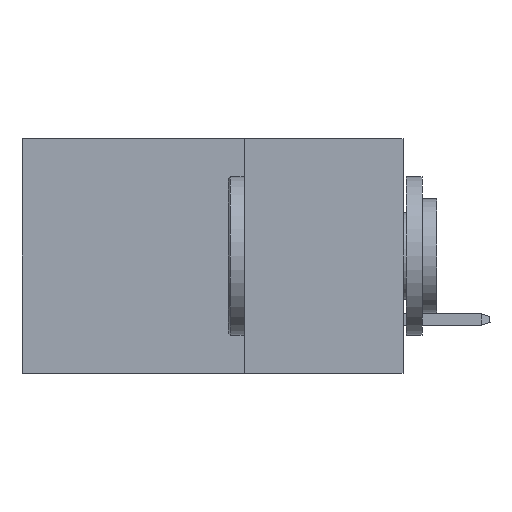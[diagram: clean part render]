
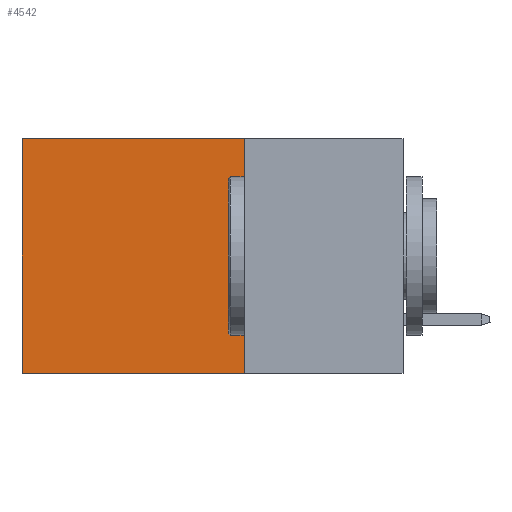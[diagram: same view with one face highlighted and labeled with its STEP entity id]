
A CAD part, left-side view. The second image highlights one B-rep face of the part: STEP entity #4542.
In plain terms, the highlighted planar face has unit normal (-1, 0, 0).
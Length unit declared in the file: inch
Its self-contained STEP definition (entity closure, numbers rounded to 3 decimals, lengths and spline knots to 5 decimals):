
#105 = VERTEX_POINT ( 'NONE', #7938 ) ;
#736 = CARTESIAN_POINT ( 'NONE',  ( 0.2875, 0.6, -0.37 ) ) ;
#773 = FACE_OUTER_BOUND ( 'NONE', #12620, .T. ) ;
#2806 = DIRECTION ( 'NONE',  ( 0., 1., 0. ) ) ;
#4542 = ADVANCED_FACE ( 'NONE', ( #773 ), #39157, .F. ) ;
#7938 = CARTESIAN_POINT ( 'NONE',  ( 0.2875, 0.25, -0.37 ) ) ;
#8342 = DIRECTION ( 'NONE',  ( 0., 0., -1. ) ) ;
#8519 = ORIENTED_EDGE ( 'NONE', *, *, #19342, .F. ) ;
#10536 = CARTESIAN_POINT ( 'NONE',  ( 0.2875, 0.25, 0. ) ) ;
#10607 = VECTOR ( 'NONE', #21859, 39.37008 ) ;
#10879 = VECTOR ( 'NONE', #2806, 39.37008 ) ;
#11262 = LINE ( 'NONE', #11458, #16919 ) ;
#11458 = CARTESIAN_POINT ( 'NONE',  ( 0.2875, 0.6, 0. ) ) ;
#12620 = EDGE_LOOP ( 'NONE', ( #39764, #29908, #8519, #24910 ) ) ;
#13743 = VERTEX_POINT ( 'NONE', #37082 ) ;
#15112 = EDGE_CURVE ( 'NONE', #27222, #13743, #31443, .T. ) ;
#15869 = EDGE_CURVE ( 'NONE', #13743, #30124, #11262, .T. ) ;
#16919 = VECTOR ( 'NONE', #8342, 39.37008 ) ;
#18236 = CARTESIAN_POINT ( 'NONE',  ( 0.2875, 0.25, 0. ) ) ;
#18391 = DIRECTION ( 'NONE',  ( 0., 0., -1. ) ) ;
#18647 = AXIS2_PLACEMENT_3D ( 'NONE', #10536, #32322, #23384 ) ;
#19342 = EDGE_CURVE ( 'NONE', #27222, #105, #33955, .T. ) ;
#21859 = DIRECTION ( 'NONE',  ( 0., 1., 0. ) ) ;
#22992 = VECTOR ( 'NONE', #18391, 39.37008 ) ;
#23158 = EDGE_CURVE ( 'NONE', #105, #30124, #37854, .T. ) ;
#23384 = DIRECTION ( 'NONE',  ( 0., 0., -1. ) ) ;
#24910 = ORIENTED_EDGE ( 'NONE', *, *, #15112, .T. ) ;
#25864 = CARTESIAN_POINT ( 'NONE',  ( 0.2875, 0.25, 0. ) ) ;
#27222 = VERTEX_POINT ( 'NONE', #18236 ) ;
#28922 = CARTESIAN_POINT ( 'NONE',  ( 0.2875, 0.25, -0.37 ) ) ;
#29908 = ORIENTED_EDGE ( 'NONE', *, *, #23158, .F. ) ;
#30124 = VERTEX_POINT ( 'NONE', #736 ) ;
#31443 = LINE ( 'NONE', #25864, #10879 ) ;
#31447 = CARTESIAN_POINT ( 'NONE',  ( 0.2875, 0.25, 0. ) ) ;
#32322 = DIRECTION ( 'NONE',  ( 1., 0., 0. ) ) ;
#33955 = LINE ( 'NONE', #31447, #22992 ) ;
#37082 = CARTESIAN_POINT ( 'NONE',  ( 0.2875, 0.6, 0. ) ) ;
#37854 = LINE ( 'NONE', #28922, #10607 ) ;
#39157 = PLANE ( 'NONE',  #18647 ) ;
#39764 = ORIENTED_EDGE ( 'NONE', *, *, #15869, .T. ) ;
